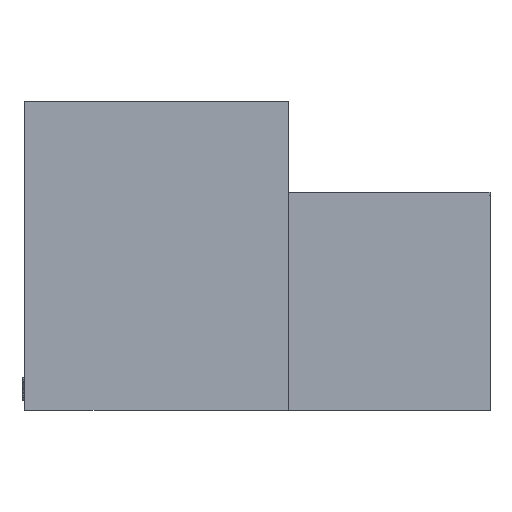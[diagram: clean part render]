
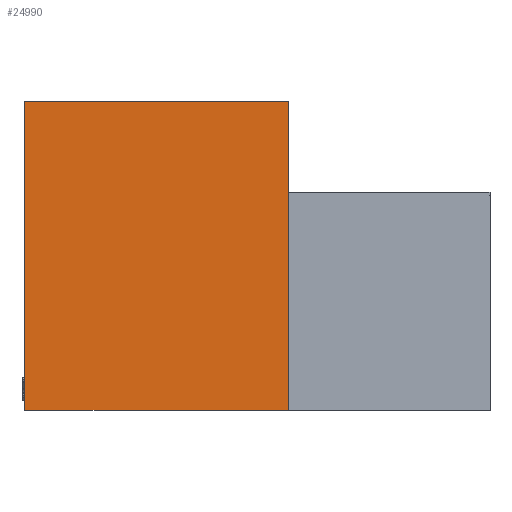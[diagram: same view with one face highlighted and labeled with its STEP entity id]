
A CAD part, left-side view. The second image highlights one B-rep face of the part: STEP entity #24990.
In plain terms, the highlighted planar face has unit normal (-1, 0, 0).
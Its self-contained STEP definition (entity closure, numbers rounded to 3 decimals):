
#524 = EDGE_CURVE ( 'NONE', #22187, #8055, #18602, .T. ) ;
#1792 = DIRECTION ( 'NONE',  ( 1., 0., 0. ) ) ;
#2571 = CARTESIAN_POINT ( 'NONE',  ( 0., 11.506, 0. ) ) ;
#4171 = CARTESIAN_POINT ( 'NONE',  ( 0., 0., -13.487 ) ) ;
#5296 = CARTESIAN_POINT ( 'NONE',  ( 0., 11.506, -13.487 ) ) ;
#6870 = CARTESIAN_POINT ( 'NONE',  ( 0., 11.506, 0. ) ) ;
#8055 = VERTEX_POINT ( 'NONE', #8812 ) ;
#8643 = ORIENTED_EDGE ( 'NONE', *, *, #25610, .F. ) ;
#8812 = CARTESIAN_POINT ( 'NONE',  ( 0., 11.506, -13.487 ) ) ;
#10272 = ORIENTED_EDGE ( 'NONE', *, *, #524, .F. ) ;
#10389 = VERTEX_POINT ( 'NONE', #2571 ) ;
#11853 = DIRECTION ( 'NONE',  ( 0., 0., -1. ) ) ;
#12055 = VECTOR ( 'NONE', #20148, 1000. ) ;
#12418 = VECTOR ( 'NONE', #23134, 1000. ) ;
#12940 = ORIENTED_EDGE ( 'NONE', *, *, #22423, .F. ) ;
#13609 = PLANE ( 'NONE',  #13795 ) ;
#13795 = AXIS2_PLACEMENT_3D ( 'NONE', #15513, #1792, #11853 ) ;
#14853 = LINE ( 'NONE', #17778, #12055 ) ;
#15205 = FACE_OUTER_BOUND ( 'NONE', #15298, .T. ) ;
#15298 = EDGE_LOOP ( 'NONE', ( #10272, #8643, #12940, #18775 ) ) ;
#15513 = CARTESIAN_POINT ( 'NONE',  ( 0., 0., 0. ) ) ;
#16045 = CARTESIAN_POINT ( 'NONE',  ( 0., -8.814, -13.487 ) ) ;
#16423 = VECTOR ( 'NONE', #18050, 1000. ) ;
#16994 = VERTEX_POINT ( 'NONE', #18206 ) ;
#17255 = DIRECTION ( 'NONE',  ( 0., 0., 1. ) ) ;
#17697 = LINE ( 'NONE', #6870, #12418 ) ;
#17778 = CARTESIAN_POINT ( 'NONE',  ( 0., 0., 0. ) ) ;
#18050 = DIRECTION ( 'NONE',  ( 0., 1., 0. ) ) ;
#18112 = EDGE_CURVE ( 'NONE', #8055, #10389, #18231, .T. ) ;
#18206 = CARTESIAN_POINT ( 'NONE',  ( 0., 0., 0. ) ) ;
#18231 = LINE ( 'NONE', #5296, #25741 ) ;
#18602 = LINE ( 'NONE', #16045, #16423 ) ;
#18775 = ORIENTED_EDGE ( 'NONE', *, *, #18112, .F. ) ;
#20148 = DIRECTION ( 'NONE',  ( 0., 0., -1. ) ) ;
#22187 = VERTEX_POINT ( 'NONE', #4171 ) ;
#22423 = EDGE_CURVE ( 'NONE', #10389, #16994, #17697, .T. ) ;
#23134 = DIRECTION ( 'NONE',  ( 0., -1., 0. ) ) ;
#24990 = ADVANCED_FACE ( 'NONE', ( #15205 ), #13609, .F. ) ;
#25610 = EDGE_CURVE ( 'NONE', #16994, #22187, #14853, .T. ) ;
#25741 = VECTOR ( 'NONE', #17255, 1000. ) ;
